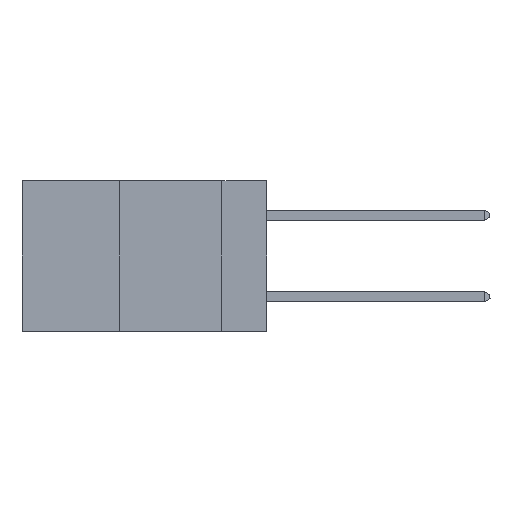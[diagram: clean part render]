
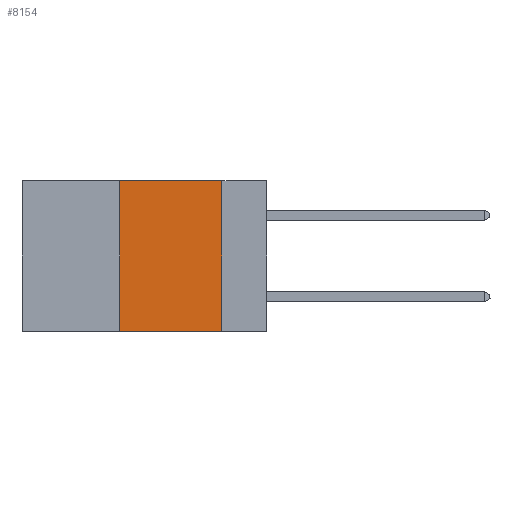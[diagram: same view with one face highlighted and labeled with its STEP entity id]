
A CAD part, left-side view. The second image highlights one B-rep face of the part: STEP entity #8154.
In plain terms, the highlighted planar face has unit normal (-1, 0, 0).
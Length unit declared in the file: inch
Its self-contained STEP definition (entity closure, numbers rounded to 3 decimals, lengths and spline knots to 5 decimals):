
#248 = DIRECTION ( 'NONE',  ( 0., 0., 1. ) ) ;
#584 = EDGE_LOOP ( 'NONE', ( #12928, #24382, #24215, #19010 ) ) ;
#3489 = VECTOR ( 'NONE', #17236, 39.37008 ) ;
#3842 = EDGE_CURVE ( 'NONE', #10036, #13878, #7463, .T. ) ;
#6432 = CARTESIAN_POINT ( 'NONE',  ( 0., 0.11, -0.37 ) ) ;
#7076 = PLANE ( 'NONE',  #9530 ) ;
#7249 = VECTOR ( 'NONE', #248, 39.37008 ) ;
#7463 = LINE ( 'NONE', #15541, #18976 ) ;
#7466 = VECTOR ( 'NONE', #17270, 39.37008 ) ;
#8154 = ADVANCED_FACE ( 'NONE', ( #19959 ), #7076, .F. ) ;
#8279 = CARTESIAN_POINT ( 'NONE',  ( 0., 0.11, 0. ) ) ;
#9530 = AXIS2_PLACEMENT_3D ( 'NONE', #11139, #15271, #23606 ) ;
#9661 = VERTEX_POINT ( 'NONE', #11428 ) ;
#10036 = VERTEX_POINT ( 'NONE', #8279 ) ;
#10794 = EDGE_CURVE ( 'NONE', #20209, #13878, #11877, .T. ) ;
#11098 = CARTESIAN_POINT ( 'NONE',  ( 0., 0.6, 0. ) ) ;
#11139 = CARTESIAN_POINT ( 'NONE',  ( 0., 0.6, 0. ) ) ;
#11428 = CARTESIAN_POINT ( 'NONE',  ( 0., 0.36, 0. ) ) ;
#11877 = LINE ( 'NONE', #18989, #3489 ) ;
#12928 = ORIENTED_EDGE ( 'NONE', *, *, #3842, .F. ) ;
#13878 = VERTEX_POINT ( 'NONE', #6432 ) ;
#15271 = DIRECTION ( 'NONE',  ( 1., 0., 0. ) ) ;
#15541 = CARTESIAN_POINT ( 'NONE',  ( 0., 0.11, 0. ) ) ;
#17236 = DIRECTION ( 'NONE',  ( 0., -1., 0. ) ) ;
#17270 = DIRECTION ( 'NONE',  ( 0., -1., 0. ) ) ;
#18310 = EDGE_CURVE ( 'NONE', #9661, #10036, #24799, .T. ) ;
#18976 = VECTOR ( 'NONE', #19776, 39.37008 ) ;
#18989 = CARTESIAN_POINT ( 'NONE',  ( 0., 0.6, -0.37 ) ) ;
#19010 = ORIENTED_EDGE ( 'NONE', *, *, #10794, .T. ) ;
#19776 = DIRECTION ( 'NONE',  ( 0., 0., -1. ) ) ;
#19959 = FACE_OUTER_BOUND ( 'NONE', #584, .T. ) ;
#20209 = VERTEX_POINT ( 'NONE', #20471 ) ;
#20471 = CARTESIAN_POINT ( 'NONE',  ( 0., 0.36, -0.37 ) ) ;
#21370 = LINE ( 'NONE', #24841, #7249 ) ;
#23606 = DIRECTION ( 'NONE',  ( 0., 0., -1. ) ) ;
#24215 = ORIENTED_EDGE ( 'NONE', *, *, #25433, .F. ) ;
#24382 = ORIENTED_EDGE ( 'NONE', *, *, #18310, .F. ) ;
#24799 = LINE ( 'NONE', #11098, #7466 ) ;
#24841 = CARTESIAN_POINT ( 'NONE',  ( 0., 0.36, 0. ) ) ;
#25433 = EDGE_CURVE ( 'NONE', #20209, #9661, #21370, .T. ) ;
